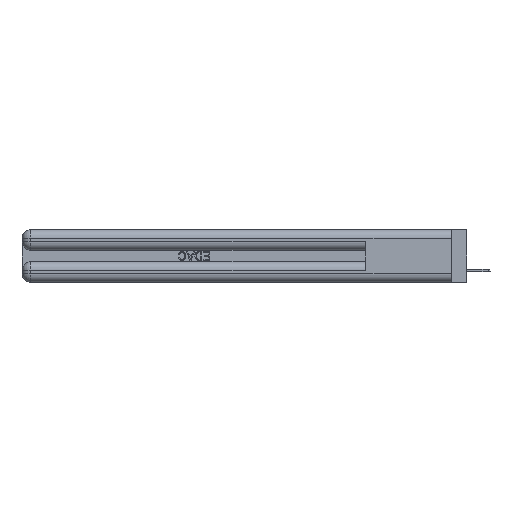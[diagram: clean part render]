
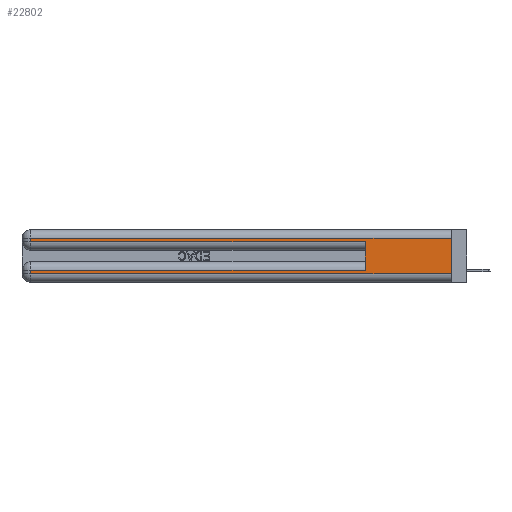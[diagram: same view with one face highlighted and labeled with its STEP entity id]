
A CAD part, left-side view. The second image highlights one B-rep face of the part: STEP entity #22802.
In plain terms, the highlighted planar face has unit normal (-1, 0, 0).
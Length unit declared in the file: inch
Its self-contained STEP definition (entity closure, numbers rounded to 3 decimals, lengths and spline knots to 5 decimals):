
#47 = DIRECTION ( 'NONE',  ( 0., 1., 0. ) ) ;
#513 = EDGE_CURVE ( 'NONE', #17481, #34381, #5449, .T. ) ;
#708 = VECTOR ( 'NONE', #4432, 39.37008 ) ;
#948 = LINE ( 'NONE', #24312, #31485 ) ;
#1208 = CARTESIAN_POINT ( 'NONE',  ( 0., 2.94, 0.085 ) ) ;
#1610 = VECTOR ( 'NONE', #16192, 39.37008 ) ;
#1891 = ORIENTED_EDGE ( 'NONE', *, *, #19864, .F. ) ;
#2860 = DIRECTION ( 'NONE',  ( 0., 0., 1. ) ) ;
#3387 = FACE_OUTER_BOUND ( 'NONE', #14375, .T. ) ;
#4432 = DIRECTION ( 'NONE',  ( 0., 0., -1. ) ) ;
#4582 = CARTESIAN_POINT ( 'NONE',  ( 0., 0.6, 0.285 ) ) ;
#5449 = LINE ( 'NONE', #27093, #25447 ) ;
#6905 = LINE ( 'NONE', #38831, #25042 ) ;
#9512 = VERTEX_POINT ( 'NONE', #1208 ) ;
#9570 = CARTESIAN_POINT ( 'NONE',  ( 0., 0.6, 0.085 ) ) ;
#10902 = EDGE_CURVE ( 'NONE', #15348, #22021, #14924, .T. ) ;
#10948 = CARTESIAN_POINT ( 'NONE',  ( 0., 2.94, 0.06 ) ) ;
#11003 = CARTESIAN_POINT ( 'NONE',  ( 0., 2.94, 0.285 ) ) ;
#12347 = VECTOR ( 'NONE', #38407, 39.37008 ) ;
#12433 = CARTESIAN_POINT ( 'NONE',  ( 0., 0., 0.31 ) ) ;
#13776 = LINE ( 'NONE', #30066, #17093 ) ;
#13846 = ORIENTED_EDGE ( 'NONE', *, *, #25395, .T. ) ;
#14031 = CARTESIAN_POINT ( 'NONE',  ( 0., 0., 0.31 ) ) ;
#14143 = CARTESIAN_POINT ( 'NONE',  ( 0., 0., 0.06 ) ) ;
#14375 = EDGE_LOOP ( 'NONE', ( #27539, #29270, #39301, #30824, #1891, #13846, #22423, #29019 ) ) ;
#14920 = DIRECTION ( 'NONE',  ( 0., 0., -1. ) ) ;
#14924 = LINE ( 'NONE', #14143, #1610 ) ;
#15348 = VERTEX_POINT ( 'NONE', #10948 ) ;
#15583 = VERTEX_POINT ( 'NONE', #12433 ) ;
#15674 = EDGE_CURVE ( 'NONE', #15583, #22021, #24159, .T. ) ;
#16192 = DIRECTION ( 'NONE',  ( 0., -1., 0. ) ) ;
#17093 = VECTOR ( 'NONE', #47, 39.37008 ) ;
#17124 = DIRECTION ( 'NONE',  ( 0., -1., 0. ) ) ;
#17323 = DIRECTION ( 'NONE',  ( 1., 0., 0. ) ) ;
#17481 = VERTEX_POINT ( 'NONE', #20318 ) ;
#18976 = EDGE_CURVE ( 'NONE', #9512, #15348, #30158, .T. ) ;
#19864 = EDGE_CURVE ( 'NONE', #32375, #30511, #948, .T. ) ;
#20313 = EDGE_CURVE ( 'NONE', #15583, #17481, #34779, .T. ) ;
#20318 = CARTESIAN_POINT ( 'NONE',  ( 0., 2.94, 0.31 ) ) ;
#22021 = VERTEX_POINT ( 'NONE', #31055 ) ;
#22423 = ORIENTED_EDGE ( 'NONE', *, *, #18976, .T. ) ;
#22802 = ADVANCED_FACE ( 'NONE', ( #3387 ), #32549, .F. ) ;
#23366 = CARTESIAN_POINT ( 'NONE',  ( 0., 0., 0.37 ) ) ;
#23504 = AXIS2_PLACEMENT_3D ( 'NONE', #23366, #17323, #39038 ) ;
#24159 = LINE ( 'NONE', #31741, #708 ) ;
#24312 = CARTESIAN_POINT ( 'NONE',  ( 0., 0.6, 0.145 ) ) ;
#25042 = VECTOR ( 'NONE', #17124, 39.37008 ) ;
#25395 = EDGE_CURVE ( 'NONE', #32375, #9512, #13776, .T. ) ;
#25447 = VECTOR ( 'NONE', #14920, 39.37008 ) ;
#27093 = CARTESIAN_POINT ( 'NONE',  ( 0., 2.94, 0.37 ) ) ;
#27539 = ORIENTED_EDGE ( 'NONE', *, *, #15674, .F. ) ;
#28629 = CARTESIAN_POINT ( 'NONE',  ( 0., 2.94, 0.37 ) ) ;
#29019 = ORIENTED_EDGE ( 'NONE', *, *, #10902, .T. ) ;
#29270 = ORIENTED_EDGE ( 'NONE', *, *, #20313, .T. ) ;
#30066 = CARTESIAN_POINT ( 'NONE',  ( 0., 0., 0.085 ) ) ;
#30158 = LINE ( 'NONE', #28629, #37804 ) ;
#30511 = VERTEX_POINT ( 'NONE', #4582 ) ;
#30824 = ORIENTED_EDGE ( 'NONE', *, *, #37143, .T. ) ;
#31055 = CARTESIAN_POINT ( 'NONE',  ( 0., 0., 0.06 ) ) ;
#31416 = DIRECTION ( 'NONE',  ( 0., 0., -1. ) ) ;
#31485 = VECTOR ( 'NONE', #2860, 39.37008 ) ;
#31741 = CARTESIAN_POINT ( 'NONE',  ( 0., 0., 0.37 ) ) ;
#32375 = VERTEX_POINT ( 'NONE', #9570 ) ;
#32549 = PLANE ( 'NONE',  #23504 ) ;
#34381 = VERTEX_POINT ( 'NONE', #11003 ) ;
#34779 = LINE ( 'NONE', #14031, #12347 ) ;
#37143 = EDGE_CURVE ( 'NONE', #34381, #30511, #6905, .T. ) ;
#37804 = VECTOR ( 'NONE', #31416, 39.37008 ) ;
#38407 = DIRECTION ( 'NONE',  ( 0., 1., 0. ) ) ;
#38831 = CARTESIAN_POINT ( 'NONE',  ( 0., 0., 0.285 ) ) ;
#39038 = DIRECTION ( 'NONE',  ( 0., 0., -1. ) ) ;
#39301 = ORIENTED_EDGE ( 'NONE', *, *, #513, .T. ) ;
